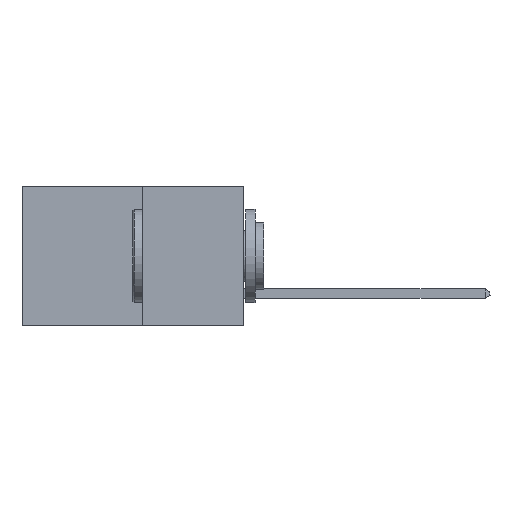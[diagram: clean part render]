
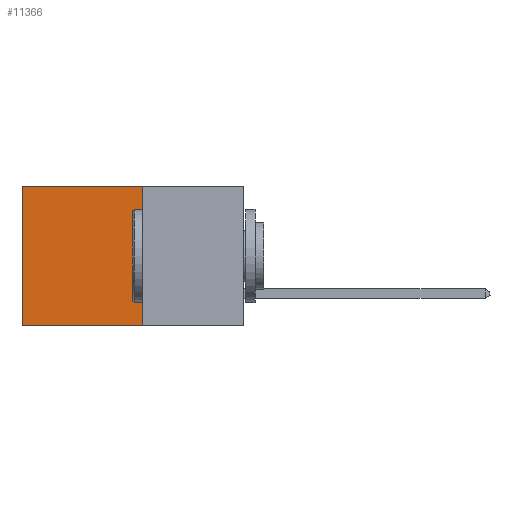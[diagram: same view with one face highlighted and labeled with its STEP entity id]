
A CAD part, left-side view. The second image highlights one B-rep face of the part: STEP entity #11366.
In plain terms, the highlighted planar face has unit normal (-1, 0, 0).
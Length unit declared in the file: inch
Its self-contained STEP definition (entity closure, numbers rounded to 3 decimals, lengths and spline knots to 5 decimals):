
#131 = VERTEX_POINT ( 'NONE', #19854 ) ;
#239 = CARTESIAN_POINT ( 'NONE',  ( 0.277, 0.59, 0. ) ) ;
#594 = CARTESIAN_POINT ( 'NONE',  ( 0.277, 0.27, -0.37 ) ) ;
#1204 = ORIENTED_EDGE ( 'NONE', *, *, #1614, .F. ) ;
#1540 = DIRECTION ( 'NONE',  ( 0., 1., 0. ) ) ;
#1614 = EDGE_CURVE ( 'NONE', #7608, #4381, #19321, .T. ) ;
#2568 = DIRECTION ( 'NONE',  ( 0., 0., -1. ) ) ;
#3247 = EDGE_CURVE ( 'NONE', #131, #7608, #6166, .T. ) ;
#4038 = CARTESIAN_POINT ( 'NONE',  ( 0.277, 0.27, -0.37 ) ) ;
#4381 = VERTEX_POINT ( 'NONE', #13029 ) ;
#4405 = VECTOR ( 'NONE', #1540, 39.37008 ) ;
#4907 = EDGE_CURVE ( 'NONE', #21107, #4381, #11134, .T. ) ;
#5787 = CARTESIAN_POINT ( 'NONE',  ( 0.277, 0.27, -0.37 ) ) ;
#6166 = LINE ( 'NONE', #11545, #15881 ) ;
#7067 = ORIENTED_EDGE ( 'NONE', *, *, #4907, .T. ) ;
#7608 = VERTEX_POINT ( 'NONE', #5787 ) ;
#7774 = FACE_OUTER_BOUND ( 'NONE', #23350, .T. ) ;
#9760 = LINE ( 'NONE', #12975, #19492 ) ;
#10900 = ORIENTED_EDGE ( 'NONE', *, *, #19462, .T. ) ;
#11134 = LINE ( 'NONE', #13168, #16273 ) ;
#11300 = DIRECTION ( 'NONE',  ( 0., 0., -1. ) ) ;
#11366 = ADVANCED_FACE ( 'NONE', ( #7774 ), #20025, .F. ) ;
#11545 = CARTESIAN_POINT ( 'NONE',  ( 0.277, 0.27, -0.37 ) ) ;
#12975 = CARTESIAN_POINT ( 'NONE',  ( 0.277, 0.27, 0. ) ) ;
#13029 = CARTESIAN_POINT ( 'NONE',  ( 0.277, 0.59, -0.37 ) ) ;
#13168 = CARTESIAN_POINT ( 'NONE',  ( 0.277, 0.59, -0.37 ) ) ;
#14269 = DIRECTION ( 'NONE',  ( 1., 0., 0. ) ) ;
#14482 = ORIENTED_EDGE ( 'NONE', *, *, #3247, .F. ) ;
#14935 = DIRECTION ( 'NONE',  ( 0., 1., 0. ) ) ;
#15210 = DIRECTION ( 'NONE',  ( 0., 0., -1. ) ) ;
#15722 = AXIS2_PLACEMENT_3D ( 'NONE', #594, #14269, #2568 ) ;
#15881 = VECTOR ( 'NONE', #11300, 39.37008 ) ;
#16273 = VECTOR ( 'NONE', #15210, 39.37008 ) ;
#19321 = LINE ( 'NONE', #4038, #4405 ) ;
#19462 = EDGE_CURVE ( 'NONE', #131, #21107, #9760, .T. ) ;
#19492 = VECTOR ( 'NONE', #14935, 39.37008 ) ;
#19854 = CARTESIAN_POINT ( 'NONE',  ( 0.277, 0.27, 0. ) ) ;
#20025 = PLANE ( 'NONE',  #15722 ) ;
#21107 = VERTEX_POINT ( 'NONE', #239 ) ;
#23350 = EDGE_LOOP ( 'NONE', ( #7067, #1204, #14482, #10900 ) ) ;
